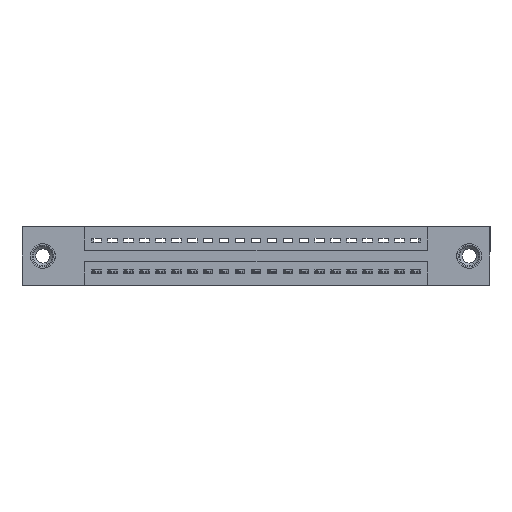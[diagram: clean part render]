
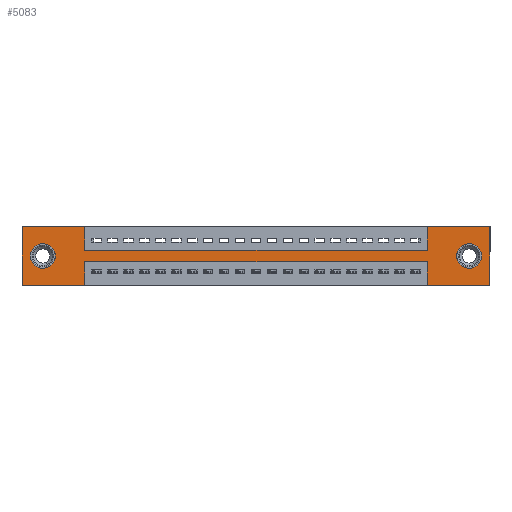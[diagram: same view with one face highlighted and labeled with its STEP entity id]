
A CAD part, front view. The second image highlights one B-rep face of the part: STEP entity #5083.
In plain terms, the highlighted planar face has unit normal (0, -1, 0).
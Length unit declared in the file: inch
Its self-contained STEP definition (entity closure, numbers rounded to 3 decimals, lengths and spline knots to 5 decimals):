
#103 = CARTESIAN_POINT ( 'NONE',  ( 2.805, 0., -0.185 ) ) ;
#234 = VERTEX_POINT ( 'NONE', #3728 ) ;
#263 = LINE ( 'NONE', #2364, #11863 ) ;
#329 = VERTEX_POINT ( 'NONE', #5923 ) ;
#352 = ORIENTED_EDGE ( 'NONE', *, *, #4777, .F. ) ;
#1000 = EDGE_CURVE ( 'NONE', #20449, #14024, #3371, .T. ) ;
#1058 = EDGE_LOOP ( 'NONE', ( #2965, #6544 ) ) ;
#1213 = CARTESIAN_POINT ( 'NONE',  ( 0., 0., 0. ) ) ;
#1419 = DIRECTION ( 'NONE',  ( -1., 0., 0. ) ) ;
#1499 = CARTESIAN_POINT ( 'NONE',  ( 2.805, 0., -0.263 ) ) ;
#1784 = CARTESIAN_POINT ( 'NONE',  ( 2.935, 0., 0. ) ) ;
#1845 = ORIENTED_EDGE ( 'NONE', *, *, #5920, .F. ) ;
#2034 = ORIENTED_EDGE ( 'NONE', *, *, #3376, .F. ) ;
#2318 = CARTESIAN_POINT ( 'NONE',  ( 0.3925, 0., -0.37 ) ) ;
#2364 = CARTESIAN_POINT ( 'NONE',  ( 2.5425, 0., -0.37 ) ) ;
#2407 = VERTEX_POINT ( 'NONE', #1499 ) ;
#2538 = CARTESIAN_POINT ( 'NONE',  ( 2.935, 0., 0. ) ) ;
#2709 = AXIS2_PLACEMENT_3D ( 'NONE', #10595, #7681, #2923 ) ;
#2718 = ORIENTED_EDGE ( 'NONE', *, *, #8143, .F. ) ;
#2743 = CARTESIAN_POINT ( 'NONE',  ( 2.5425, 0., 0. ) ) ;
#2798 = VECTOR ( 'NONE', #10074, 39.37008 ) ;
#2853 = ORIENTED_EDGE ( 'NONE', *, *, #4427, .T. ) ;
#2923 = DIRECTION ( 'NONE',  ( 0., 0., -1. ) ) ;
#2936 = ORIENTED_EDGE ( 'NONE', *, *, #1000, .F. ) ;
#2965 = ORIENTED_EDGE ( 'NONE', *, *, #4476, .T. ) ;
#3033 = CIRCLE ( 'NONE', #7815, 0.078 ) ;
#3075 = CARTESIAN_POINT ( 'NONE',  ( 0.13, 0., -0.185 ) ) ;
#3116 = VECTOR ( 'NONE', #4658, 39.37008 ) ;
#3219 = DIRECTION ( 'NONE',  ( 0., 0., 1. ) ) ;
#3255 = LINE ( 'NONE', #17830, #10295 ) ;
#3371 = LINE ( 'NONE', #1213, #3116 ) ;
#3376 = EDGE_CURVE ( 'NONE', #5657, #10620, #19429, .T. ) ;
#3720 = EDGE_CURVE ( 'NONE', #6901, #5657, #15875, .T. ) ;
#3728 = CARTESIAN_POINT ( 'NONE',  ( 2.5425, 0., -0.37 ) ) ;
#3793 = DIRECTION ( 'NONE',  ( 0., 0., -1. ) ) ;
#3920 = CARTESIAN_POINT ( 'NONE',  ( 0.3925, 0., -0.15 ) ) ;
#4427 = EDGE_CURVE ( 'NONE', #2407, #17271, #18909, .T. ) ;
#4476 = EDGE_CURVE ( 'NONE', #9081, #7497, #12401, .T. ) ;
#4549 = CARTESIAN_POINT ( 'NONE',  ( 0., 0., -0.37 ) ) ;
#4571 = VECTOR ( 'NONE', #9314, 39.37008 ) ;
#4632 = VECTOR ( 'NONE', #19196, 39.37008 ) ;
#4658 = DIRECTION ( 'NONE',  ( 0., 0., 1. ) ) ;
#4777 = EDGE_CURVE ( 'NONE', #234, #17371, #263, .T. ) ;
#4852 = EDGE_CURVE ( 'NONE', #329, #234, #13098, .T. ) ;
#4860 = LINE ( 'NONE', #2318, #13127 ) ;
#4961 = ORIENTED_EDGE ( 'NONE', *, *, #14323, .F. ) ;
#5083 = ADVANCED_FACE ( 'NONE', ( #11329, #18875, #11845 ), #8957, .T. ) ;
#5252 = CARTESIAN_POINT ( 'NONE',  ( 0., 0., 0. ) ) ;
#5582 = CARTESIAN_POINT ( 'NONE',  ( 0.3925, 0., -0.37 ) ) ;
#5657 = VERTEX_POINT ( 'NONE', #3920 ) ;
#5762 = CARTESIAN_POINT ( 'NONE',  ( 0.13, 0., -0.107 ) ) ;
#5920 = EDGE_CURVE ( 'NONE', #18237, #18246, #10790, .T. ) ;
#5923 = CARTESIAN_POINT ( 'NONE',  ( 2.935, 0., -0.37 ) ) ;
#6037 = CARTESIAN_POINT ( 'NONE',  ( 0., 0., -0.37 ) ) ;
#6173 = DIRECTION ( 'NONE',  ( 0., 0., -1. ) ) ;
#6305 = ORIENTED_EDGE ( 'NONE', *, *, #8331, .T. ) ;
#6543 = CARTESIAN_POINT ( 'NONE',  ( 0.3925, 0., 0. ) ) ;
#6544 = ORIENTED_EDGE ( 'NONE', *, *, #19877, .T. ) ;
#6655 = ORIENTED_EDGE ( 'NONE', *, *, #3720, .F. ) ;
#6724 = DIRECTION ( 'NONE',  ( 0., 0., 1. ) ) ;
#6764 = LINE ( 'NONE', #1784, #2798 ) ;
#6883 = CARTESIAN_POINT ( 'NONE',  ( 2.805, 0., -0.107 ) ) ;
#6901 = VERTEX_POINT ( 'NONE', #6543 ) ;
#7091 = VECTOR ( 'NONE', #14916, 39.37008 ) ;
#7497 = VERTEX_POINT ( 'NONE', #16908 ) ;
#7681 = DIRECTION ( 'NONE',  ( 0., -1., 0. ) ) ;
#7815 = AXIS2_PLACEMENT_3D ( 'NONE', #8468, #13395, #3793 ) ;
#8046 = LINE ( 'NONE', #5252, #18619 ) ;
#8143 = EDGE_CURVE ( 'NONE', #14024, #6901, #8046, .T. ) ;
#8331 = EDGE_CURVE ( 'NONE', #17271, #2407, #3033, .T. ) ;
#8468 = CARTESIAN_POINT ( 'NONE',  ( 2.805, 0., -0.185 ) ) ;
#8957 = PLANE ( 'NONE',  #2709 ) ;
#9081 = VERTEX_POINT ( 'NONE', #5762 ) ;
#9132 = EDGE_CURVE ( 'NONE', #13537, #20449, #3255, .T. ) ;
#9270 = AXIS2_PLACEMENT_3D ( 'NONE', #103, #13053, #11368 ) ;
#9314 = DIRECTION ( 'NONE',  ( -1., 0., 0. ) ) ;
#9340 = CARTESIAN_POINT ( 'NONE',  ( 0.3925, 0., -0.22 ) ) ;
#9642 = CARTESIAN_POINT ( 'NONE',  ( 0.3925, 0., 0. ) ) ;
#9722 = ORIENTED_EDGE ( 'NONE', *, *, #9132, .F. ) ;
#10074 = DIRECTION ( 'NONE',  ( 0., 0., -1. ) ) ;
#10295 = VECTOR ( 'NONE', #17982, 39.37008 ) ;
#10406 = LINE ( 'NONE', #9340, #18427 ) ;
#10458 = VERTEX_POINT ( 'NONE', #13280 ) ;
#10514 = CARTESIAN_POINT ( 'NONE',  ( 0., 0., 0. ) ) ;
#10595 = CARTESIAN_POINT ( 'NONE',  ( 0., 0., -0.37 ) ) ;
#10620 = VERTEX_POINT ( 'NONE', #12636 ) ;
#10790 = LINE ( 'NONE', #10514, #13558 ) ;
#11039 = AXIS2_PLACEMENT_3D ( 'NONE', #12360, #20400, #19010 ) ;
#11326 = ORIENTED_EDGE ( 'NONE', *, *, #12349, .F. ) ;
#11329 = FACE_BOUND ( 'NONE', #19799, .T. ) ;
#11368 = DIRECTION ( 'NONE',  ( 0., 0., -1. ) ) ;
#11508 = CARTESIAN_POINT ( 'NONE',  ( 0.3925, 0., -0.15 ) ) ;
#11845 = FACE_OUTER_BOUND ( 'NONE', #15819, .T. ) ;
#11863 = VECTOR ( 'NONE', #6724, 39.37008 ) ;
#12037 = CARTESIAN_POINT ( 'NONE',  ( 2.5425, 0., 0. ) ) ;
#12286 = CARTESIAN_POINT ( 'NONE',  ( 2.5425, 0., -0.22 ) ) ;
#12349 = EDGE_CURVE ( 'NONE', #17371, #10458, #10406, .T. ) ;
#12360 = CARTESIAN_POINT ( 'NONE',  ( 0.13, 0., -0.185 ) ) ;
#12401 = CIRCLE ( 'NONE', #11039, 0.078 ) ;
#12636 = CARTESIAN_POINT ( 'NONE',  ( 2.5425, 0., -0.15 ) ) ;
#13053 = DIRECTION ( 'NONE',  ( 0., 1., 0. ) ) ;
#13098 = LINE ( 'NONE', #6037, #4571 ) ;
#13127 = VECTOR ( 'NONE', #6173, 39.37008 ) ;
#13169 = CARTESIAN_POINT ( 'NONE',  ( 0., 0., 0. ) ) ;
#13280 = CARTESIAN_POINT ( 'NONE',  ( 0.3925, 0., -0.22 ) ) ;
#13395 = DIRECTION ( 'NONE',  ( 0., 1., 0. ) ) ;
#13453 = ORIENTED_EDGE ( 'NONE', *, *, #4852, .F. ) ;
#13537 = VERTEX_POINT ( 'NONE', #5582 ) ;
#13558 = VECTOR ( 'NONE', #15375, 39.37008 ) ;
#14024 = VERTEX_POINT ( 'NONE', #13169 ) ;
#14173 = DIRECTION ( 'NONE',  ( 0., 0., 1. ) ) ;
#14323 = EDGE_CURVE ( 'NONE', #10458, #13537, #4860, .T. ) ;
#14411 = ORIENTED_EDGE ( 'NONE', *, *, #15179, .F. ) ;
#14916 = DIRECTION ( 'NONE',  ( 1., 0., 0. ) ) ;
#15150 = CIRCLE ( 'NONE', #18478, 0.078 ) ;
#15179 = EDGE_CURVE ( 'NONE', #10620, #18237, #15812, .T. ) ;
#15261 = EDGE_CURVE ( 'NONE', #18246, #329, #6764, .T. ) ;
#15324 = VECTOR ( 'NONE', #14173, 39.37008 ) ;
#15375 = DIRECTION ( 'NONE',  ( 1., 0., 0. ) ) ;
#15812 = LINE ( 'NONE', #12037, #15324 ) ;
#15819 = EDGE_LOOP ( 'NONE', ( #4961, #11326, #352, #13453, #17010, #1845, #14411, #2034, #6655, #2718, #2936, #9722 ) ) ;
#15875 = LINE ( 'NONE', #9642, #4632 ) ;
#16296 = DIRECTION ( 'NONE',  ( 1., 0., 0. ) ) ;
#16908 = CARTESIAN_POINT ( 'NONE',  ( 0.13, 0., -0.263 ) ) ;
#17010 = ORIENTED_EDGE ( 'NONE', *, *, #15261, .F. ) ;
#17271 = VERTEX_POINT ( 'NONE', #6883 ) ;
#17371 = VERTEX_POINT ( 'NONE', #12286 ) ;
#17830 = CARTESIAN_POINT ( 'NONE',  ( 0., 0., -0.37 ) ) ;
#17982 = DIRECTION ( 'NONE',  ( -1., 0., 0. ) ) ;
#18237 = VERTEX_POINT ( 'NONE', #2743 ) ;
#18246 = VERTEX_POINT ( 'NONE', #2538 ) ;
#18427 = VECTOR ( 'NONE', #1419, 39.37008 ) ;
#18478 = AXIS2_PLACEMENT_3D ( 'NONE', #3075, #20830, #3219 ) ;
#18619 = VECTOR ( 'NONE', #16296, 39.37008 ) ;
#18875 = FACE_BOUND ( 'NONE', #1058, .T. ) ;
#18909 = CIRCLE ( 'NONE', #9270, 0.078 ) ;
#19010 = DIRECTION ( 'NONE',  ( 0., 0., 1. ) ) ;
#19196 = DIRECTION ( 'NONE',  ( 0., 0., -1. ) ) ;
#19429 = LINE ( 'NONE', #11508, #7091 ) ;
#19799 = EDGE_LOOP ( 'NONE', ( #6305, #2853 ) ) ;
#19877 = EDGE_CURVE ( 'NONE', #7497, #9081, #15150, .T. ) ;
#20400 = DIRECTION ( 'NONE',  ( 0., 1., 0. ) ) ;
#20449 = VERTEX_POINT ( 'NONE', #4549 ) ;
#20830 = DIRECTION ( 'NONE',  ( 0., 1., 0. ) ) ;
